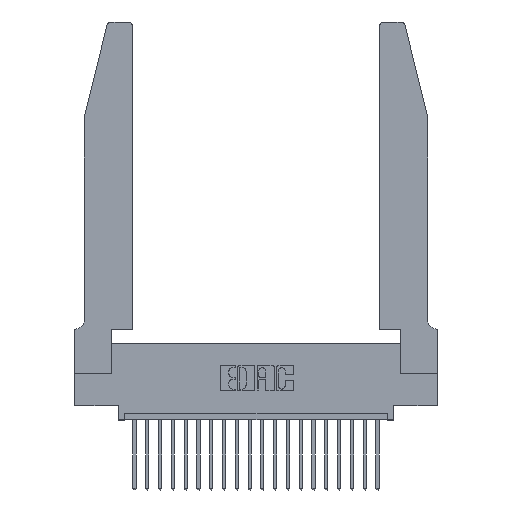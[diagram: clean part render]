
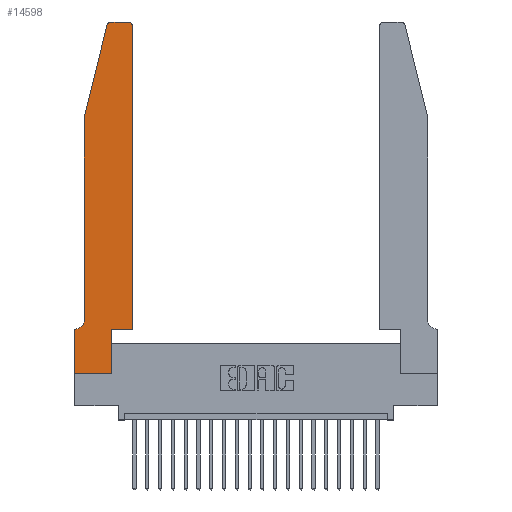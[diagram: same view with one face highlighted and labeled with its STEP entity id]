
A CAD part, top view. The second image highlights one B-rep face of the part: STEP entity #14598.
In plain terms, the highlighted planar face has unit normal (0, 0, 1).
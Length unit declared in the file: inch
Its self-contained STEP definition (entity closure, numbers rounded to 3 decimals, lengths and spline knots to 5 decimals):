
#9 = DIRECTION ( 'NONE',  ( 0., -1., 0. ) ) ;
#134 = AXIS2_PLACEMENT_3D ( 'NONE', #22729, #19585, #7025 ) ;
#938 = DIRECTION ( 'NONE',  ( 1., 0., 0. ) ) ;
#1116 = LINE ( 'NONE', #22271, #9419 ) ;
#1621 = DIRECTION ( 'NONE',  ( 1., 0., 0. ) ) ;
#2286 = CIRCLE ( 'NONE', #20502, 0.07 ) ;
#2320 = CARTESIAN_POINT ( 'NONE',  ( 0., 0., 0.37 ) ) ;
#2330 = DIRECTION ( 'NONE',  ( 0., -1., 0. ) ) ;
#2960 = CARTESIAN_POINT ( 'NONE',  ( 0.4205, 2.72, 0.37 ) ) ;
#3214 = PLANE ( 'NONE',  #134 ) ;
#3742 = CARTESIAN_POINT ( 'NONE',  ( 0.0755, 0.42, 0.37 ) ) ;
#3783 = CARTESIAN_POINT ( 'NONE',  ( 0., 0.35, 0.37 ) ) ;
#3922 = DIRECTION ( 'NONE',  ( -1., 0., 0. ) ) ;
#4019 = CARTESIAN_POINT ( 'NONE',  ( 0.284, 2.75, 0.37 ) ) ;
#4050 = EDGE_CURVE ( 'NONE', #11198, #20338, #20015, .T. ) ;
#4214 = EDGE_CURVE ( 'NONE', #4522, #19183, #2286, .T. ) ;
#4448 = FACE_OUTER_BOUND ( 'NONE', #16095, .T. ) ;
#4522 = VERTEX_POINT ( 'NONE', #3742 ) ;
#4674 = DIRECTION ( 'NONE',  ( -0.239, -0.971, 0. ) ) ;
#4767 = VECTOR ( 'NONE', #8052, 39.37008 ) ;
#5732 = VERTEX_POINT ( 'NONE', #11657 ) ;
#6184 = VECTOR ( 'NONE', #9, 39.37008 ) ;
#6252 = ORIENTED_EDGE ( 'NONE', *, *, #22504, .T. ) ;
#6428 = LINE ( 'NONE', #10094, #4767 ) ;
#6827 = VERTEX_POINT ( 'NONE', #2320 ) ;
#7025 = DIRECTION ( 'NONE',  ( 1., 0., 0. ) ) ;
#7088 = EDGE_CURVE ( 'NONE', #19183, #20065, #15958, .T. ) ;
#7122 = VERTEX_POINT ( 'NONE', #8465 ) ;
#7162 = ORIENTED_EDGE ( 'NONE', *, *, #4214, .T. ) ;
#7171 = ORIENTED_EDGE ( 'NONE', *, *, #7667, .T. ) ;
#7242 = LINE ( 'NONE', #7593, #12525 ) ;
#7593 = CARTESIAN_POINT ( 'NONE',  ( 0.2865, 0.35, 0.37 ) ) ;
#7630 = AXIS2_PLACEMENT_3D ( 'NONE', #2960, #20259, #17239 ) ;
#7667 = EDGE_CURVE ( 'NONE', #16482, #5732, #13714, .T. ) ;
#7718 = ORIENTED_EDGE ( 'NONE', *, *, #14874, .T. ) ;
#7837 = EDGE_CURVE ( 'NONE', #9729, #8845, #9690, .T. ) ;
#8052 = DIRECTION ( 'NONE',  ( 0., 1., 0. ) ) ;
#8082 = EDGE_CURVE ( 'NONE', #7122, #9729, #7242, .T. ) ;
#8434 = EDGE_CURVE ( 'NONE', #8845, #16482, #6428, .T. ) ;
#8465 = CARTESIAN_POINT ( 'NONE',  ( 0.2865, 0., 0.37 ) ) ;
#8613 = VECTOR ( 'NONE', #1621, 39.37008 ) ;
#8845 = VERTEX_POINT ( 'NONE', #14034 ) ;
#9285 = ORIENTED_EDGE ( 'NONE', *, *, #18281, .T. ) ;
#9365 = ORIENTED_EDGE ( 'NONE', *, *, #7088, .T. ) ;
#9419 = VECTOR ( 'NONE', #4674, 39.37008 ) ;
#9435 = CARTESIAN_POINT ( 'NONE',  ( 0.0755, 2., 0.37 ) ) ;
#9690 = LINE ( 'NONE', #11326, #20216 ) ;
#9709 = CARTESIAN_POINT ( 'NONE',  ( 0.2865, 0.35, 0.37 ) ) ;
#9729 = VERTEX_POINT ( 'NONE', #9709 ) ;
#10086 = CARTESIAN_POINT ( 'NONE',  ( 0.284, 2.72, 0.37 ) ) ;
#10094 = CARTESIAN_POINT ( 'NONE',  ( 0.4505, 0.35, 0.37 ) ) ;
#10278 = LINE ( 'NONE', #19559, #8613 ) ;
#10591 = EDGE_CURVE ( 'NONE', #20338, #21728, #1116, .T. ) ;
#11198 = VERTEX_POINT ( 'NONE', #4019 ) ;
#11205 = EDGE_CURVE ( 'NONE', #21728, #4522, #17409, .T. ) ;
#11326 = CARTESIAN_POINT ( 'NONE',  ( 0.4505, 0.35, 0.37 ) ) ;
#11544 = DIRECTION ( 'NONE',  ( 1., 0., 0. ) ) ;
#11595 = VECTOR ( 'NONE', #12734, 39.37008 ) ;
#11657 = CARTESIAN_POINT ( 'NONE',  ( 0.4205, 2.75, 0.37 ) ) ;
#12085 = CARTESIAN_POINT ( 'NONE',  ( 0.4505, 2.72, 0.37 ) ) ;
#12275 = LINE ( 'NONE', #14223, #6184 ) ;
#12327 = CARTESIAN_POINT ( 'NONE',  ( 0.0055, 0.42, 0.37 ) ) ;
#12336 = ORIENTED_EDGE ( 'NONE', *, *, #8434, .T. ) ;
#12525 = VECTOR ( 'NONE', #14955, 39.37008 ) ;
#12592 = CARTESIAN_POINT ( 'NONE',  ( 0.2605, 2.75, 0.37 ) ) ;
#12734 = DIRECTION ( 'NONE',  ( -1., 0., 0. ) ) ;
#13714 = CIRCLE ( 'NONE', #7630, 0.03 ) ;
#14002 = DIRECTION ( 'NONE',  ( 0., 0., -1. ) ) ;
#14018 = CARTESIAN_POINT ( 'NONE',  ( 0.0755, 0.35, 0.37 ) ) ;
#14034 = CARTESIAN_POINT ( 'NONE',  ( 0.4505, 0.35, 0.37 ) ) ;
#14223 = CARTESIAN_POINT ( 'NONE',  ( 0., 0., 0.37 ) ) ;
#14598 = ADVANCED_FACE ( 'NONE', ( #4448 ), #3214, .T. ) ;
#14604 = VECTOR ( 'NONE', #2330, 39.37008 ) ;
#14874 = EDGE_CURVE ( 'NONE', #5732, #11198, #17968, .T. ) ;
#14955 = DIRECTION ( 'NONE',  ( 0., 1., 0. ) ) ;
#15101 = ORIENTED_EDGE ( 'NONE', *, *, #10591, .T. ) ;
#15267 = ORIENTED_EDGE ( 'NONE', *, *, #11205, .T. ) ;
#15945 = ORIENTED_EDGE ( 'NONE', *, *, #4050, .T. ) ;
#15958 = LINE ( 'NONE', #14018, #17628 ) ;
#16095 = EDGE_LOOP ( 'NONE', ( #7718, #15945, #15101, #15267, #7162, #9365, #6252, #9285, #20750, #22195, #12336, #7171 ) ) ;
#16304 = AXIS2_PLACEMENT_3D ( 'NONE', #10086, #17114, #938 ) ;
#16482 = VERTEX_POINT ( 'NONE', #12085 ) ;
#17114 = DIRECTION ( 'NONE',  ( 0., 0., 1. ) ) ;
#17218 = CARTESIAN_POINT ( 'NONE',  ( 0.0755, 2., 0.37 ) ) ;
#17239 = DIRECTION ( 'NONE',  ( 1., 0., 0. ) ) ;
#17409 = LINE ( 'NONE', #9435, #14604 ) ;
#17628 = VECTOR ( 'NONE', #3922, 39.37008 ) ;
#17968 = LINE ( 'NONE', #12592, #11595 ) ;
#18281 = EDGE_CURVE ( 'NONE', #6827, #7122, #10278, .T. ) ;
#18841 = CARTESIAN_POINT ( 'NONE',  ( 0.25487, 2.72718, 0.37 ) ) ;
#19183 = VERTEX_POINT ( 'NONE', #20836 ) ;
#19460 = DIRECTION ( 'NONE',  ( -1., 0., 0. ) ) ;
#19559 = CARTESIAN_POINT ( 'NONE',  ( 0., 0., 0.37 ) ) ;
#19585 = DIRECTION ( 'NONE',  ( 0., 0., 1. ) ) ;
#20015 = CIRCLE ( 'NONE', #16304, 0.03 ) ;
#20065 = VERTEX_POINT ( 'NONE', #3783 ) ;
#20216 = VECTOR ( 'NONE', #11544, 39.37008 ) ;
#20259 = DIRECTION ( 'NONE',  ( 0., 0., 1. ) ) ;
#20338 = VERTEX_POINT ( 'NONE', #18841 ) ;
#20502 = AXIS2_PLACEMENT_3D ( 'NONE', #12327, #14002, #19460 ) ;
#20750 = ORIENTED_EDGE ( 'NONE', *, *, #8082, .T. ) ;
#20836 = CARTESIAN_POINT ( 'NONE',  ( 0.0055, 0.35, 0.37 ) ) ;
#21728 = VERTEX_POINT ( 'NONE', #17218 ) ;
#22195 = ORIENTED_EDGE ( 'NONE', *, *, #7837, .T. ) ;
#22271 = CARTESIAN_POINT ( 'NONE',  ( 0.0755, 2., 0.37 ) ) ;
#22504 = EDGE_CURVE ( 'NONE', #20065, #6827, #12275, .T. ) ;
#22729 = CARTESIAN_POINT ( 'NONE',  ( 0., 0.35, 0.37 ) ) ;
